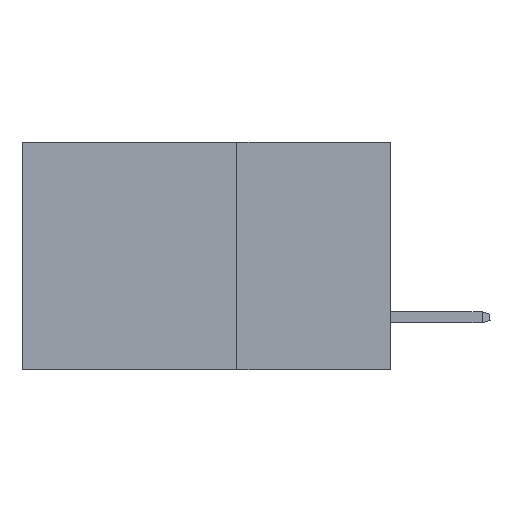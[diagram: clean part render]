
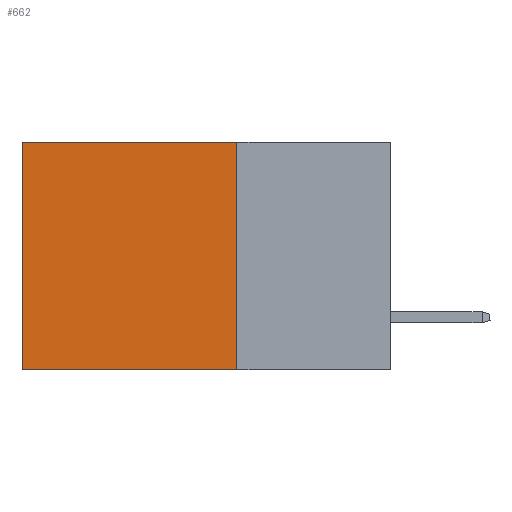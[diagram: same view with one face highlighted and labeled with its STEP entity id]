
A CAD part, left-side view. The second image highlights one B-rep face of the part: STEP entity #662.
In plain terms, the highlighted planar face has unit normal (-1, 0, 0).
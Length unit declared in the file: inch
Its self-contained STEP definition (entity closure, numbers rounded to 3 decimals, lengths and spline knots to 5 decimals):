
#662 = ADVANCED_FACE ( 'NONE', ( #26229 ), #15178, .F. ) ;
#1618 = ORIENTED_EDGE ( 'NONE', *, *, #9265, .T. ) ;
#2686 = CARTESIAN_POINT ( 'NONE',  ( 0.2875, 0.6, 0. ) ) ;
#3059 = CARTESIAN_POINT ( 'NONE',  ( 0.2875, 0.6, 0. ) ) ;
#3954 = CARTESIAN_POINT ( 'NONE',  ( 0.2875, 0.25, 0. ) ) ;
#4035 = CARTESIAN_POINT ( 'NONE',  ( 0.2875, 0.25, 0. ) ) ;
#4515 = VERTEX_POINT ( 'NONE', #26506 ) ;
#4777 = VERTEX_POINT ( 'NONE', #9611 ) ;
#5500 = LINE ( 'NONE', #4035, #12570 ) ;
#5993 = EDGE_CURVE ( 'NONE', #17014, #4515, #21032, .T. ) ;
#6577 = VECTOR ( 'NONE', #20803, 39.37008 ) ;
#8219 = DIRECTION ( 'NONE',  ( 0., 1., 0. ) ) ;
#8485 = DIRECTION ( 'NONE',  ( 0., 0., -1. ) ) ;
#8775 = VECTOR ( 'NONE', #21719, 39.37008 ) ;
#9265 = EDGE_CURVE ( 'NONE', #12604, #4515, #29231, .T. ) ;
#9611 = CARTESIAN_POINT ( 'NONE',  ( 0.2875, 0.25, 0. ) ) ;
#10177 = EDGE_CURVE ( 'NONE', #4777, #17014, #5500, .T. ) ;
#12338 = LINE ( 'NONE', #25887, #25048 ) ;
#12570 = VECTOR ( 'NONE', #28809, 39.37008 ) ;
#12604 = VERTEX_POINT ( 'NONE', #3059 ) ;
#15178 = PLANE ( 'NONE',  #27284 ) ;
#16211 = EDGE_LOOP ( 'NONE', ( #1618, #21654, #22820, #27398 ) ) ;
#17014 = VERTEX_POINT ( 'NONE', #24900 ) ;
#17437 = DIRECTION ( 'NONE',  ( 1., 0., 0. ) ) ;
#20803 = DIRECTION ( 'NONE',  ( 0., 1., 0. ) ) ;
#20996 = CARTESIAN_POINT ( 'NONE',  ( 0.2875, 0.25, -0.37 ) ) ;
#21032 = LINE ( 'NONE', #20996, #6577 ) ;
#21654 = ORIENTED_EDGE ( 'NONE', *, *, #5993, .F. ) ;
#21719 = DIRECTION ( 'NONE',  ( 0., 0., -1. ) ) ;
#22820 = ORIENTED_EDGE ( 'NONE', *, *, #10177, .F. ) ;
#24168 = EDGE_CURVE ( 'NONE', #4777, #12604, #12338, .T. ) ;
#24900 = CARTESIAN_POINT ( 'NONE',  ( 0.2875, 0.25, -0.37 ) ) ;
#25048 = VECTOR ( 'NONE', #8219, 39.37008 ) ;
#25887 = CARTESIAN_POINT ( 'NONE',  ( 0.2875, 0.25, 0. ) ) ;
#26229 = FACE_OUTER_BOUND ( 'NONE', #16211, .T. ) ;
#26506 = CARTESIAN_POINT ( 'NONE',  ( 0.2875, 0.6, -0.37 ) ) ;
#27284 = AXIS2_PLACEMENT_3D ( 'NONE', #3954, #17437, #8485 ) ;
#27398 = ORIENTED_EDGE ( 'NONE', *, *, #24168, .T. ) ;
#28809 = DIRECTION ( 'NONE',  ( 0., 0., -1. ) ) ;
#29231 = LINE ( 'NONE', #2686, #8775 ) ;
